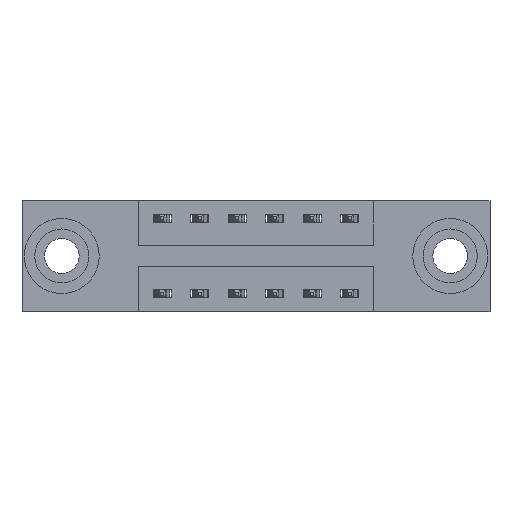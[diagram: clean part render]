
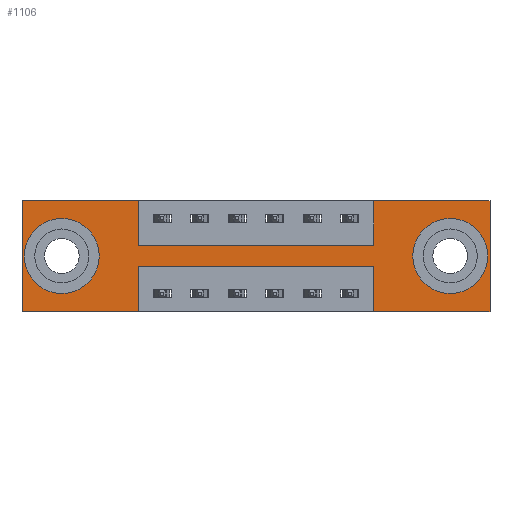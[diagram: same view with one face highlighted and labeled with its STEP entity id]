
A CAD part, front view. The second image highlights one B-rep face of the part: STEP entity #1106.
In plain terms, the highlighted planar face has unit normal (0, -1, 0).
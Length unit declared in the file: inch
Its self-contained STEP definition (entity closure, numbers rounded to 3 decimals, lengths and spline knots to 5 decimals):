
#105 = FACE_OUTER_BOUND ( 'NONE', #3213, .T. ) ;
#177 = CARTESIAN_POINT ( 'NONE',  ( 1.4275, 0., -0.263 ) ) ;
#187 = EDGE_CURVE ( 'NONE', #7718, #2888, #8661, .T. ) ;
#320 = ORIENTED_EDGE ( 'NONE', *, *, #187, .F. ) ;
#410 = PLANE ( 'NONE',  #1704 ) ;
#456 = ORIENTED_EDGE ( 'NONE', *, *, #5571, .T. ) ;
#486 = VERTEX_POINT ( 'NONE', #5791 ) ;
#499 = CARTESIAN_POINT ( 'NONE',  ( 1.4275, 0., -0.185 ) ) ;
#513 = DIRECTION ( 'NONE',  ( 0., 0., 1. ) ) ;
#536 = ORIENTED_EDGE ( 'NONE', *, *, #6892, .F. ) ;
#566 = DIRECTION ( 'NONE',  ( 1., 0., 0. ) ) ;
#591 = VERTEX_POINT ( 'NONE', #3933 ) ;
#681 = CARTESIAN_POINT ( 'NONE',  ( 0., 0., -0.37 ) ) ;
#722 = ORIENTED_EDGE ( 'NONE', *, *, #4884, .T. ) ;
#771 = CARTESIAN_POINT ( 'NONE',  ( 0., 0., 0. ) ) ;
#798 = CARTESIAN_POINT ( 'NONE',  ( 1.1725, 0., -0.15 ) ) ;
#813 = ORIENTED_EDGE ( 'NONE', *, *, #1049, .F. ) ;
#879 = VECTOR ( 'NONE', #566, 39.37008 ) ;
#1028 = DIRECTION ( 'NONE',  ( 0., 0., 1. ) ) ;
#1049 = EDGE_CURVE ( 'NONE', #3209, #2010, #9319, .T. ) ;
#1105 = CIRCLE ( 'NONE', #4854, 0.078 ) ;
#1106 = ADVANCED_FACE ( 'NONE', ( #5260, #3771, #105 ), #410, .T. ) ;
#1231 = CARTESIAN_POINT ( 'NONE',  ( 1.4275, 0., -0.107 ) ) ;
#1325 = VERTEX_POINT ( 'NONE', #7104 ) ;
#1359 = LINE ( 'NONE', #2111, #4562 ) ;
#1440 = DIRECTION ( 'NONE',  ( 0., -1., 0. ) ) ;
#1464 = CARTESIAN_POINT ( 'NONE',  ( 1.4275, 0., -0.185 ) ) ;
#1602 = DIRECTION ( 'NONE',  ( -1., 0., 0. ) ) ;
#1649 = EDGE_CURVE ( 'NONE', #4320, #486, #9109, .T. ) ;
#1704 = AXIS2_PLACEMENT_3D ( 'NONE', #681, #1440, #4464 ) ;
#1781 = LINE ( 'NONE', #2739, #5979 ) ;
#1854 = CIRCLE ( 'NONE', #6520, 0.078 ) ;
#1934 = ORIENTED_EDGE ( 'NONE', *, *, #2941, .F. ) ;
#1966 = EDGE_CURVE ( 'NONE', #9420, #7718, #4675, .T. ) ;
#2010 = VERTEX_POINT ( 'NONE', #9368 ) ;
#2024 = CARTESIAN_POINT ( 'NONE',  ( 0.3875, 0., -0.15 ) ) ;
#2035 = CIRCLE ( 'NONE', #5057, 0.078 ) ;
#2078 = DIRECTION ( 'NONE',  ( 0., 0., -1. ) ) ;
#2111 = CARTESIAN_POINT ( 'NONE',  ( 0., 0., 0. ) ) ;
#2135 = LINE ( 'NONE', #2024, #879 ) ;
#2171 = CARTESIAN_POINT ( 'NONE',  ( 0.3875, 0., -0.37 ) ) ;
#2263 = VERTEX_POINT ( 'NONE', #2942 ) ;
#2276 = DIRECTION ( 'NONE',  ( 0., 0., -1. ) ) ;
#2343 = VERTEX_POINT ( 'NONE', #1231 ) ;
#2349 = ORIENTED_EDGE ( 'NONE', *, *, #7605, .T. ) ;
#2477 = DIRECTION ( 'NONE',  ( 0., 1., 0. ) ) ;
#2634 = CARTESIAN_POINT ( 'NONE',  ( 1.1725, 0., -0.37 ) ) ;
#2690 = VERTEX_POINT ( 'NONE', #177 ) ;
#2716 = VECTOR ( 'NONE', #5046, 39.37008 ) ;
#2739 = CARTESIAN_POINT ( 'NONE',  ( 0., 0., 0. ) ) ;
#2765 = ORIENTED_EDGE ( 'NONE', *, *, #8726, .F. ) ;
#2816 = EDGE_CURVE ( 'NONE', #5661, #3209, #1781, .T. ) ;
#2888 = VERTEX_POINT ( 'NONE', #8582 ) ;
#2941 = EDGE_CURVE ( 'NONE', #591, #4320, #3322, .T. ) ;
#2942 = CARTESIAN_POINT ( 'NONE',  ( 1.1725, 0., 0. ) ) ;
#3082 = VECTOR ( 'NONE', #6100, 39.37008 ) ;
#3209 = VERTEX_POINT ( 'NONE', #3376 ) ;
#3213 = EDGE_LOOP ( 'NONE', ( #1934, #5110, #7928, #320, #4837, #536, #2765, #5564, #813, #7023, #9260, #4957 ) ) ;
#3230 = EDGE_LOOP ( 'NONE', ( #2349, #722 ) ) ;
#3322 = LINE ( 'NONE', #8791, #7108 ) ;
#3374 = CARTESIAN_POINT ( 'NONE',  ( 1.56, 0., 0. ) ) ;
#3376 = CARTESIAN_POINT ( 'NONE',  ( 0.3875, 0., 0. ) ) ;
#3391 = LINE ( 'NONE', #3552, #6851 ) ;
#3482 = CARTESIAN_POINT ( 'NONE',  ( 1.56, 0., 0. ) ) ;
#3552 = CARTESIAN_POINT ( 'NONE',  ( 1.1725, 0., 0. ) ) ;
#3771 = FACE_BOUND ( 'NONE', #6688, .T. ) ;
#3868 = VECTOR ( 'NONE', #7165, 39.37008 ) ;
#3933 = CARTESIAN_POINT ( 'NONE',  ( 0.3875, 0., -0.22 ) ) ;
#3998 = LINE ( 'NONE', #2634, #9001 ) ;
#4098 = VECTOR ( 'NONE', #2078, 39.37008 ) ;
#4320 = VERTEX_POINT ( 'NONE', #2171 ) ;
#4324 = DIRECTION ( 'NONE',  ( 0., 0., 1. ) ) ;
#4419 = LINE ( 'NONE', #771, #6152 ) ;
#4464 = DIRECTION ( 'NONE',  ( 0., 0., -1. ) ) ;
#4562 = VECTOR ( 'NONE', #4324, 39.37008 ) ;
#4662 = CARTESIAN_POINT ( 'NONE',  ( 0.1325, 0., -0.185 ) ) ;
#4675 = LINE ( 'NONE', #3482, #2716 ) ;
#4757 = EDGE_CURVE ( 'NONE', #2888, #1325, #3998, .T. ) ;
#4837 = ORIENTED_EDGE ( 'NONE', *, *, #1966, .F. ) ;
#4854 = AXIS2_PLACEMENT_3D ( 'NONE', #499, #9219, #5647 ) ;
#4884 = EDGE_CURVE ( 'NONE', #2690, #2343, #1854, .T. ) ;
#4957 = ORIENTED_EDGE ( 'NONE', *, *, #1649, .F. ) ;
#4958 = CARTESIAN_POINT ( 'NONE',  ( 0.1325, 0., -0.107 ) ) ;
#4985 = EDGE_CURVE ( 'NONE', #1325, #591, #8989, .T. ) ;
#5046 = DIRECTION ( 'NONE',  ( 0., 0., -1. ) ) ;
#5057 = AXIS2_PLACEMENT_3D ( 'NONE', #4662, #5387, #1028 ) ;
#5085 = VERTEX_POINT ( 'NONE', #798 ) ;
#5110 = ORIENTED_EDGE ( 'NONE', *, *, #4985, .F. ) ;
#5126 = CARTESIAN_POINT ( 'NONE',  ( 0., 0., -0.37 ) ) ;
#5189 = DIRECTION ( 'NONE',  ( 0., 0., -1. ) ) ;
#5260 = FACE_BOUND ( 'NONE', #3230, .T. ) ;
#5322 = EDGE_CURVE ( 'NONE', #486, #5661, #1359, .T. ) ;
#5387 = DIRECTION ( 'NONE',  ( 0., 1., 0. ) ) ;
#5540 = CARTESIAN_POINT ( 'NONE',  ( 1.56, 0., -0.37 ) ) ;
#5564 = ORIENTED_EDGE ( 'NONE', *, *, #6611, .F. ) ;
#5571 = EDGE_CURVE ( 'NONE', #6539, #8968, #2035, .T. ) ;
#5647 = DIRECTION ( 'NONE',  ( 0., 0., -1. ) ) ;
#5661 = VERTEX_POINT ( 'NONE', #5669 ) ;
#5669 = CARTESIAN_POINT ( 'NONE',  ( 0., 0., 0. ) ) ;
#5791 = CARTESIAN_POINT ( 'NONE',  ( 0., 0., -0.37 ) ) ;
#5979 = VECTOR ( 'NONE', #8557, 39.37008 ) ;
#6100 = DIRECTION ( 'NONE',  ( -1., 0., 0. ) ) ;
#6152 = VECTOR ( 'NONE', #8870, 39.37008 ) ;
#6520 = AXIS2_PLACEMENT_3D ( 'NONE', #1464, #8008, #5189 ) ;
#6526 = CARTESIAN_POINT ( 'NONE',  ( 0., 0., -0.37 ) ) ;
#6539 = VERTEX_POINT ( 'NONE', #4958 ) ;
#6611 = EDGE_CURVE ( 'NONE', #2010, #5085, #2135, .T. ) ;
#6688 = EDGE_LOOP ( 'NONE', ( #456, #9062 ) ) ;
#6851 = VECTOR ( 'NONE', #9336, 39.37008 ) ;
#6856 = CARTESIAN_POINT ( 'NONE',  ( 0.1325, 0., -0.185 ) ) ;
#6892 = EDGE_CURVE ( 'NONE', #2263, #9420, #4419, .T. ) ;
#6910 = EDGE_CURVE ( 'NONE', #8968, #6539, #7286, .T. ) ;
#7023 = ORIENTED_EDGE ( 'NONE', *, *, #2816, .F. ) ;
#7075 = AXIS2_PLACEMENT_3D ( 'NONE', #6856, #2477, #7589 ) ;
#7104 = CARTESIAN_POINT ( 'NONE',  ( 1.1725, 0., -0.22 ) ) ;
#7108 = VECTOR ( 'NONE', #2276, 39.37008 ) ;
#7165 = DIRECTION ( 'NONE',  ( -1., 0., 0. ) ) ;
#7286 = CIRCLE ( 'NONE', #7075, 0.078 ) ;
#7589 = DIRECTION ( 'NONE',  ( 0., 0., 1. ) ) ;
#7605 = EDGE_CURVE ( 'NONE', #2343, #2690, #1105, .T. ) ;
#7718 = VERTEX_POINT ( 'NONE', #5540 ) ;
#7928 = ORIENTED_EDGE ( 'NONE', *, *, #4757, .F. ) ;
#8008 = DIRECTION ( 'NONE',  ( 0., 1., 0. ) ) ;
#8455 = CARTESIAN_POINT ( 'NONE',  ( 0.3875, 0., -0.22 ) ) ;
#8557 = DIRECTION ( 'NONE',  ( 1., 0., 0. ) ) ;
#8582 = CARTESIAN_POINT ( 'NONE',  ( 1.1725, 0., -0.37 ) ) ;
#8654 = CARTESIAN_POINT ( 'NONE',  ( 0.3875, 0., 0. ) ) ;
#8661 = LINE ( 'NONE', #5126, #3082 ) ;
#8726 = EDGE_CURVE ( 'NONE', #5085, #2263, #3391, .T. ) ;
#8791 = CARTESIAN_POINT ( 'NONE',  ( 0.3875, 0., -0.37 ) ) ;
#8870 = DIRECTION ( 'NONE',  ( 1., 0., 0. ) ) ;
#8968 = VERTEX_POINT ( 'NONE', #9092 ) ;
#8989 = LINE ( 'NONE', #8455, #9110 ) ;
#9001 = VECTOR ( 'NONE', #513, 39.37008 ) ;
#9062 = ORIENTED_EDGE ( 'NONE', *, *, #6910, .T. ) ;
#9092 = CARTESIAN_POINT ( 'NONE',  ( 0.1325, 0., -0.263 ) ) ;
#9109 = LINE ( 'NONE', #6526, #3868 ) ;
#9110 = VECTOR ( 'NONE', #1602, 39.37008 ) ;
#9219 = DIRECTION ( 'NONE',  ( 0., 1., 0. ) ) ;
#9260 = ORIENTED_EDGE ( 'NONE', *, *, #5322, .F. ) ;
#9319 = LINE ( 'NONE', #8654, #4098 ) ;
#9336 = DIRECTION ( 'NONE',  ( 0., 0., 1. ) ) ;
#9368 = CARTESIAN_POINT ( 'NONE',  ( 0.3875, 0., -0.15 ) ) ;
#9420 = VERTEX_POINT ( 'NONE', #3374 ) ;
